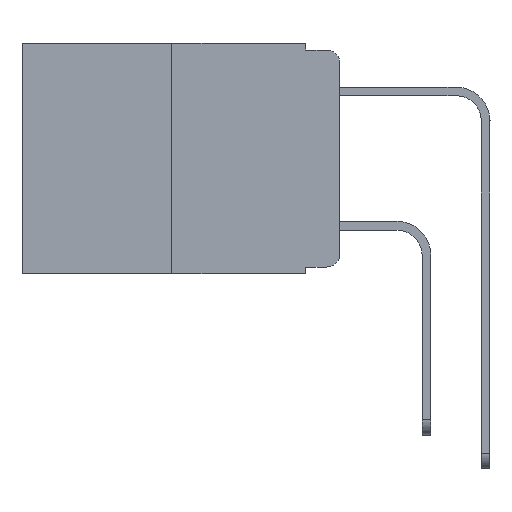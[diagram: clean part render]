
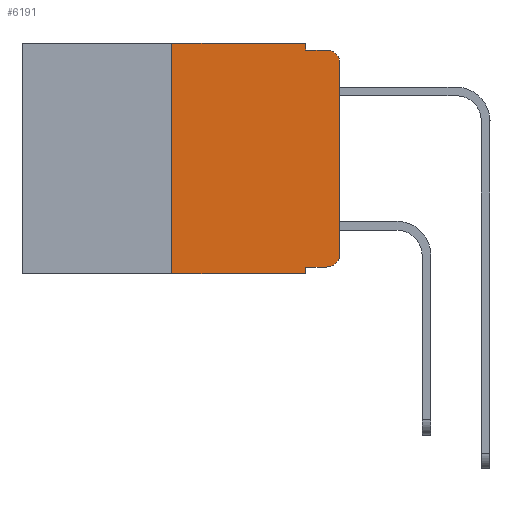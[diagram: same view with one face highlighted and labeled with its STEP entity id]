
A CAD part, left-side view. The second image highlights one B-rep face of the part: STEP entity #6191.
In plain terms, the highlighted planar face has unit normal (-1, 0, 0).
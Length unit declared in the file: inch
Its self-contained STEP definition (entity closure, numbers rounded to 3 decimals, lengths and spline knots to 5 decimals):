
#261 = ORIENTED_EDGE ( 'NONE', *, *, #6387, .T. ) ;
#390 = DIRECTION ( 'NONE',  ( 0., -1., 0. ) ) ;
#535 = DIRECTION ( 'NONE',  ( 0., 0., -1. ) ) ;
#636 = CARTESIAN_POINT ( 'NONE',  ( 0., 0.02, -0.03 ) ) ;
#681 = AXIS2_PLACEMENT_3D ( 'NONE', #8803, #9210, #4101 ) ;
#818 = VECTOR ( 'NONE', #12408, 39.37008 ) ;
#863 = AXIS2_PLACEMENT_3D ( 'NONE', #12833, #10689, #535 ) ;
#1273 = ORIENTED_EDGE ( 'NONE', *, *, #1541, .F. ) ;
#1541 = EDGE_CURVE ( 'NONE', #2509, #6672, #11262, .T. ) ;
#1913 = VERTEX_POINT ( 'NONE', #7792 ) ;
#2368 = VERTEX_POINT ( 'NONE', #4353 ) ;
#2509 = VERTEX_POINT ( 'NONE', #12245 ) ;
#2797 = CARTESIAN_POINT ( 'NONE',  ( 0., 0.25, 0. ) ) ;
#2876 = CARTESIAN_POINT ( 'NONE',  ( 0., 0., -0.03 ) ) ;
#2896 = EDGE_LOOP ( 'NONE', ( #11348, #5631, #8067, #4945, #7103, #1273, #6766, #6490, #10244, #261 ) ) ;
#2993 = LINE ( 'NONE', #9459, #5576 ) ;
#3336 = VERTEX_POINT ( 'NONE', #2876 ) ;
#4101 = DIRECTION ( 'NONE',  ( 0., 0., -1. ) ) ;
#4353 = CARTESIAN_POINT ( 'NONE',  ( 0., 0.051, -0.343 ) ) ;
#4420 = CARTESIAN_POINT ( 'NONE',  ( 0., 0.051, 0. ) ) ;
#4603 = VECTOR ( 'NONE', #13402, 39.37008 ) ;
#4616 = DIRECTION ( 'NONE',  ( 0., -1., 0. ) ) ;
#4945 = ORIENTED_EDGE ( 'NONE', *, *, #6751, .F. ) ;
#5183 = LINE ( 'NONE', #6725, #10390 ) ;
#5307 = DIRECTION ( 'NONE',  ( 0., -1., 0. ) ) ;
#5576 = VECTOR ( 'NONE', #5307, 39.37008 ) ;
#5631 = ORIENTED_EDGE ( 'NONE', *, *, #7958, .T. ) ;
#5773 = VERTEX_POINT ( 'NONE', #9650 ) ;
#5775 = LINE ( 'NONE', #12289, #6428 ) ;
#5857 = VECTOR ( 'NONE', #7699, 39.37008 ) ;
#6023 = DIRECTION ( 'NONE',  ( 0., 0., -1. ) ) ;
#6191 = ADVANCED_FACE ( 'NONE', ( #9324 ), #10821, .F. ) ;
#6387 = EDGE_CURVE ( 'NONE', #1913, #12086, #9207, .T. ) ;
#6428 = VECTOR ( 'NONE', #390, 39.37008 ) ;
#6490 = ORIENTED_EDGE ( 'NONE', *, *, #10462, .F. ) ;
#6672 = VERTEX_POINT ( 'NONE', #2797 ) ;
#6725 = CARTESIAN_POINT ( 'NONE',  ( 0., 0.473, 0. ) ) ;
#6751 = EDGE_CURVE ( 'NONE', #8492, #7576, #10162, .T. ) ;
#6766 = ORIENTED_EDGE ( 'NONE', *, *, #10124, .T. ) ;
#6984 = CARTESIAN_POINT ( 'NONE',  ( 0., 0.051, -0.01 ) ) ;
#7103 = ORIENTED_EDGE ( 'NONE', *, *, #9906, .F. ) ;
#7323 = EDGE_CURVE ( 'NONE', #7576, #9105, #5775, .T. ) ;
#7561 = AXIS2_PLACEMENT_3D ( 'NONE', #636, #12879, #6023 ) ;
#7576 = VERTEX_POINT ( 'NONE', #6984 ) ;
#7678 = EDGE_CURVE ( 'NONE', #12086, #3336, #8226, .T. ) ;
#7699 = DIRECTION ( 'NONE',  ( 0., 0., 1. ) ) ;
#7792 = CARTESIAN_POINT ( 'NONE',  ( 0., 0.02, -0.333 ) ) ;
#7809 = CARTESIAN_POINT ( 'NONE',  ( 0., 0., -0.313 ) ) ;
#7948 = DIRECTION ( 'NONE',  ( 0., 0., 1. ) ) ;
#7951 = CARTESIAN_POINT ( 'NONE',  ( 0., 0., 0. ) ) ;
#7958 = EDGE_CURVE ( 'NONE', #3336, #9105, #9829, .T. ) ;
#8067 = ORIENTED_EDGE ( 'NONE', *, *, #7323, .F. ) ;
#8226 = LINE ( 'NONE', #7951, #9993 ) ;
#8492 = VERTEX_POINT ( 'NONE', #4420 ) ;
#8803 = CARTESIAN_POINT ( 'NONE',  ( 0., 0.02, -0.313 ) ) ;
#8884 = EDGE_CURVE ( 'NONE', #5773, #1913, #2993, .T. ) ;
#9105 = VERTEX_POINT ( 'NONE', #12809 ) ;
#9207 = CIRCLE ( 'NONE', #681, 0.02 ) ;
#9210 = DIRECTION ( 'NONE',  ( -1., 0., 0. ) ) ;
#9240 = CARTESIAN_POINT ( 'NONE',  ( 0., 0.473, -0.343 ) ) ;
#9324 = FACE_OUTER_BOUND ( 'NONE', #2896, .T. ) ;
#9421 = LINE ( 'NONE', #10563, #818 ) ;
#9459 = CARTESIAN_POINT ( 'NONE',  ( 0., 0.051, -0.333 ) ) ;
#9579 = LINE ( 'NONE', #9240, #11824 ) ;
#9650 = CARTESIAN_POINT ( 'NONE',  ( 0., 0.051, -0.333 ) ) ;
#9829 = CIRCLE ( 'NONE', #7561, 0.02 ) ;
#9906 = EDGE_CURVE ( 'NONE', #6672, #8492, #5183, .T. ) ;
#9993 = VECTOR ( 'NONE', #7948, 39.37008 ) ;
#10124 = EDGE_CURVE ( 'NONE', #2509, #2368, #9579, .T. ) ;
#10162 = LINE ( 'NONE', #12566, #4603 ) ;
#10244 = ORIENTED_EDGE ( 'NONE', *, *, #8884, .T. ) ;
#10275 = DIRECTION ( 'NONE',  ( 0., -1., 0. ) ) ;
#10390 = VECTOR ( 'NONE', #4616, 39.37008 ) ;
#10462 = EDGE_CURVE ( 'NONE', #5773, #2368, #9421, .T. ) ;
#10563 = CARTESIAN_POINT ( 'NONE',  ( 0., 0.051, 0. ) ) ;
#10689 = DIRECTION ( 'NONE',  ( 1., 0., 0. ) ) ;
#10821 = PLANE ( 'NONE',  #863 ) ;
#11262 = LINE ( 'NONE', #12950, #5857 ) ;
#11348 = ORIENTED_EDGE ( 'NONE', *, *, #7678, .T. ) ;
#11824 = VECTOR ( 'NONE', #10275, 39.37008 ) ;
#12086 = VERTEX_POINT ( 'NONE', #7809 ) ;
#12245 = CARTESIAN_POINT ( 'NONE',  ( 0., 0.25, -0.343 ) ) ;
#12289 = CARTESIAN_POINT ( 'NONE',  ( 0., 0.051, -0.01 ) ) ;
#12408 = DIRECTION ( 'NONE',  ( 0., 0., -1. ) ) ;
#12566 = CARTESIAN_POINT ( 'NONE',  ( 0., 0.051, 0. ) ) ;
#12809 = CARTESIAN_POINT ( 'NONE',  ( 0., 0.02, -0.01 ) ) ;
#12833 = CARTESIAN_POINT ( 'NONE',  ( 0., 0.473, 0. ) ) ;
#12879 = DIRECTION ( 'NONE',  ( -1., 0., 0. ) ) ;
#12950 = CARTESIAN_POINT ( 'NONE',  ( 0., 0.25, 0. ) ) ;
#13402 = DIRECTION ( 'NONE',  ( 0., 0., -1. ) ) ;
